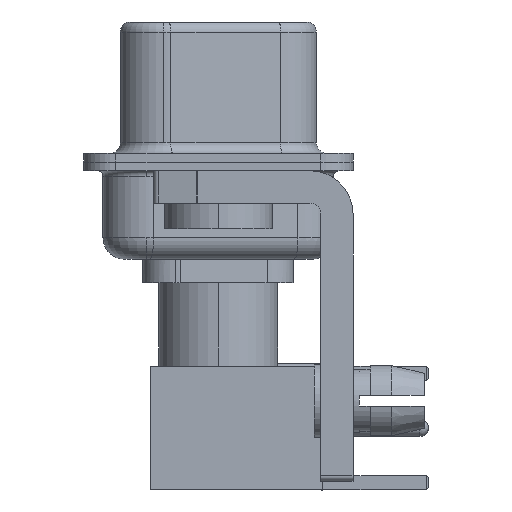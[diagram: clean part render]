
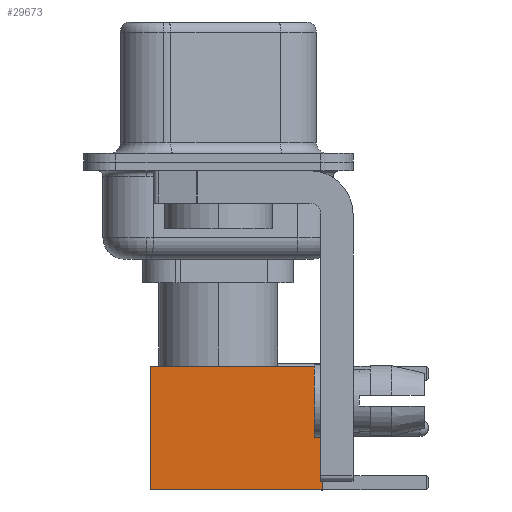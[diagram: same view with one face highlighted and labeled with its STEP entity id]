
A CAD part, left-side view. The second image highlights one B-rep face of the part: STEP entity #29673.
In plain terms, the highlighted face is planar.
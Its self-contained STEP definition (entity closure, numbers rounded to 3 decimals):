
#63 = CARTESIAN_POINT ( 'NONE',  ( 2.875, 2.875, 0. ) ) ;
#2770 = PLANE ( 'NONE',  #32733 ) ;
#3115 = DIRECTION ( 'NONE',  ( 0., 0., 1. ) ) ;
#4201 = DIRECTION ( 'NONE',  ( -1., 0., 0. ) ) ;
#5333 = ORIENTED_EDGE ( 'NONE', *, *, #33550, .T. ) ;
#5425 = CARTESIAN_POINT ( 'NONE',  ( -2.875, 2.875, 8. ) ) ;
#5798 = CARTESIAN_POINT ( 'NONE',  ( 2.875, 2.875, 0. ) ) ;
#6629 = VECTOR ( 'NONE', #18462, 1000. ) ;
#8082 = DIRECTION ( 'NONE',  ( -1., 0., 0. ) ) ;
#8285 = ORIENTED_EDGE ( 'NONE', *, *, #14504, .T. ) ;
#8641 = DIRECTION ( 'NONE',  ( 0., 1., 0. ) ) ;
#12405 = ORIENTED_EDGE ( 'NONE', *, *, #24059, .F. ) ;
#13288 = VECTOR ( 'NONE', #24802, 1000. ) ;
#13321 = VERTEX_POINT ( 'NONE', #5425 ) ;
#13680 = CARTESIAN_POINT ( 'NONE',  ( -2.875, 2.875, 0. ) ) ;
#14504 = EDGE_CURVE ( 'NONE', #29876, #20436, #28895, .T. ) ;
#15565 = EDGE_CURVE ( 'NONE', #13321, #31738, #32594, .T. ) ;
#18462 = DIRECTION ( 'NONE',  ( 0., 0., -1. ) ) ;
#18643 = CARTESIAN_POINT ( 'NONE',  ( 0., 2.875, 8. ) ) ;
#20436 = VERTEX_POINT ( 'NONE', #63 ) ;
#21988 = VECTOR ( 'NONE', #8082, 1000. ) ;
#22578 = LINE ( 'NONE', #30223, #25764 ) ;
#24059 = EDGE_CURVE ( 'NONE', #29876, #13321, #26469, .T. ) ;
#24440 = FACE_OUTER_BOUND ( 'NONE', #27605, .T. ) ;
#24714 = ORIENTED_EDGE ( 'NONE', *, *, #15565, .F. ) ;
#24802 = DIRECTION ( 'NONE',  ( 0., 0., -1. ) ) ;
#25764 = VECTOR ( 'NONE', #4201, 1000. ) ;
#26305 = CARTESIAN_POINT ( 'NONE',  ( -2.875, 2.875, 0. ) ) ;
#26469 = LINE ( 'NONE', #18643, #21988 ) ;
#27605 = EDGE_LOOP ( 'NONE', ( #8285, #5333, #24714, #12405 ) ) ;
#28895 = LINE ( 'NONE', #5798, #6629 ) ;
#29673 = ADVANCED_FACE ( 'NONE', ( #24440 ), #2770, .T. ) ;
#29876 = VERTEX_POINT ( 'NONE', #30337 ) ;
#30223 = CARTESIAN_POINT ( 'NONE',  ( 0., 2.875, 0. ) ) ;
#30337 = CARTESIAN_POINT ( 'NONE',  ( 2.875, 2.875, 8. ) ) ;
#31738 = VERTEX_POINT ( 'NONE', #26305 ) ;
#31891 = CARTESIAN_POINT ( 'NONE',  ( 2.875, 2.875, 0. ) ) ;
#32594 = LINE ( 'NONE', #13680, #13288 ) ;
#32733 = AXIS2_PLACEMENT_3D ( 'NONE', #31891, #8641, #3115 ) ;
#33550 = EDGE_CURVE ( 'NONE', #20436, #31738, #22578, .T. ) ;
